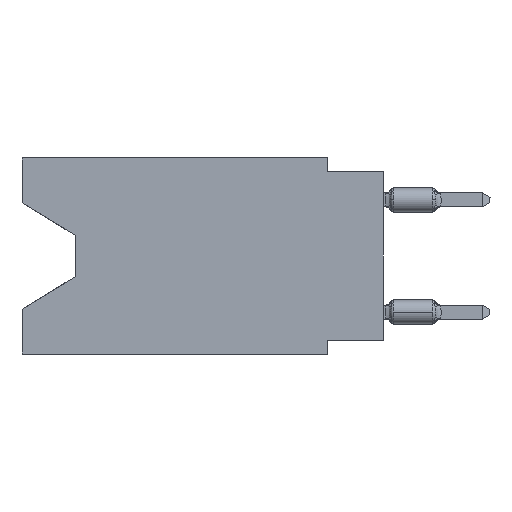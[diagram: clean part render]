
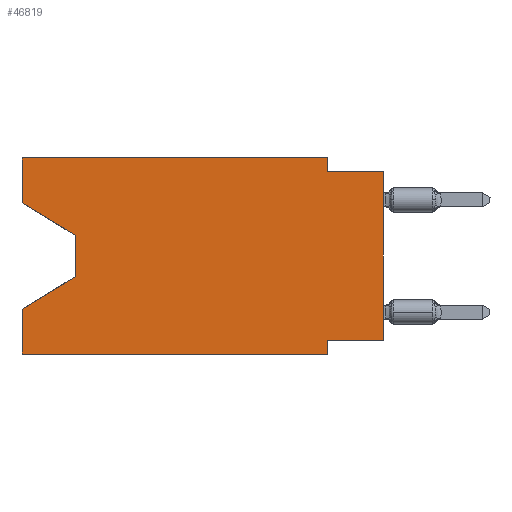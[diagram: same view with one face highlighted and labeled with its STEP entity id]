
A CAD part, left-side view. The second image highlights one B-rep face of the part: STEP entity #46819.
In plain terms, the highlighted planar face has unit normal (-1, 0, 0).
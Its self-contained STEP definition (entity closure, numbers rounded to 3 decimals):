
#721 = CARTESIAN_POINT ( 'NONE',  ( 0., 13.97, -5.385 ) ) ;
#1086 = EDGE_CURVE ( 'NONE', #20945, #19968, #5221, .T. ) ;
#1559 = CARTESIAN_POINT ( 'NONE',  ( 0., 16.383, -2.038 ) ) ;
#1664 = EDGE_CURVE ( 'NONE', #19952, #47622, #46606, .T. ) ;
#1917 = VECTOR ( 'NONE', #2793, 1000. ) ;
#2793 = DIRECTION ( 'NONE',  ( 0., 1., 0. ) ) ;
#3804 = CARTESIAN_POINT ( 'NONE',  ( 0., 16.383, 0. ) ) ;
#3839 = DIRECTION ( 'NONE',  ( 0., 0., -1. ) ) ;
#4248 = FACE_OUTER_BOUND ( 'NONE', #30074, .T. ) ;
#4250 = ORIENTED_EDGE ( 'NONE', *, *, #1664, .F. ) ;
#4386 = CARTESIAN_POINT ( 'NONE',  ( 0., 2.54, -8.255 ) ) ;
#4581 = VECTOR ( 'NONE', #15181, 1000. ) ;
#4975 = CARTESIAN_POINT ( 'NONE',  ( 0., 16.383, -2.038 ) ) ;
#5157 = ORIENTED_EDGE ( 'NONE', *, *, #45447, .F. ) ;
#5221 = LINE ( 'NONE', #34377, #26325 ) ;
#5437 = LINE ( 'NONE', #12619, #23388 ) ;
#5651 = ORIENTED_EDGE ( 'NONE', *, *, #29624, .F. ) ;
#6024 = VECTOR ( 'NONE', #39168, 1000. ) ;
#6646 = CARTESIAN_POINT ( 'NONE',  ( 0., 0., -8.255 ) ) ;
#7120 = CARTESIAN_POINT ( 'NONE',  ( 0., 16.383, -6.852 ) ) ;
#7619 = LINE ( 'NONE', #34495, #47470 ) ;
#7646 = DIRECTION ( 'NONE',  ( 0., -1., 0. ) ) ;
#9174 = LINE ( 'NONE', #24790, #21552 ) ;
#10894 = ORIENTED_EDGE ( 'NONE', *, *, #1086, .F. ) ;
#11537 = CARTESIAN_POINT ( 'NONE',  ( 0., 16.383, -8.89 ) ) ;
#12569 = DIRECTION ( 'NONE',  ( 0., -0.855, -0.519 ) ) ;
#12619 = CARTESIAN_POINT ( 'NONE',  ( 0., 16.383, -8.89 ) ) ;
#12793 = CARTESIAN_POINT ( 'NONE',  ( 0., 13.97, -5.385 ) ) ;
#13985 = ORIENTED_EDGE ( 'NONE', *, *, #17828, .T. ) ;
#15181 = DIRECTION ( 'NONE',  ( 0., 0., 1. ) ) ;
#15222 = VERTEX_POINT ( 'NONE', #11537 ) ;
#15249 = DIRECTION ( 'NONE',  ( 1., 0., 0. ) ) ;
#15275 = EDGE_CURVE ( 'NONE', #15731, #26305, #31252, .T. ) ;
#15731 = VERTEX_POINT ( 'NONE', #721 ) ;
#17105 = ORIENTED_EDGE ( 'NONE', *, *, #17678, .F. ) ;
#17678 = EDGE_CURVE ( 'NONE', #15222, #26305, #27218, .T. ) ;
#17828 = EDGE_CURVE ( 'NONE', #15222, #47622, #5437, .T. ) ;
#18212 = CARTESIAN_POINT ( 'NONE',  ( 0., 0., -0.635 ) ) ;
#18218 = ORIENTED_EDGE ( 'NONE', *, *, #15275, .T. ) ;
#18248 = ORIENTED_EDGE ( 'NONE', *, *, #48105, .F. ) ;
#19952 = VERTEX_POINT ( 'NONE', #4386 ) ;
#19968 = VERTEX_POINT ( 'NONE', #42783 ) ;
#20094 = EDGE_CURVE ( 'NONE', #20945, #23039, #44067, .T. ) ;
#20847 = CARTESIAN_POINT ( 'NONE',  ( 0., 2.54, 0. ) ) ;
#20945 = VERTEX_POINT ( 'NONE', #4975 ) ;
#21552 = VECTOR ( 'NONE', #47845, 1000. ) ;
#22370 = VECTOR ( 'NONE', #12569, 1000. ) ;
#23039 = VERTEX_POINT ( 'NONE', #49503 ) ;
#23190 = VECTOR ( 'NONE', #42718, 1000. ) ;
#23388 = VECTOR ( 'NONE', #24413, 1000. ) ;
#24151 = CARTESIAN_POINT ( 'NONE',  ( 0., 2.54, -0.635 ) ) ;
#24413 = DIRECTION ( 'NONE',  ( 0., -1., 0. ) ) ;
#24699 = LINE ( 'NONE', #20847, #35748 ) ;
#24790 = CARTESIAN_POINT ( 'NONE',  ( 0., 0., 0. ) ) ;
#24795 = VECTOR ( 'NONE', #3839, 1000. ) ;
#25985 = VERTEX_POINT ( 'NONE', #18212 ) ;
#26107 = LINE ( 'NONE', #6646, #1917 ) ;
#26305 = VERTEX_POINT ( 'NONE', #7120 ) ;
#26325 = VECTOR ( 'NONE', #38208, 1000. ) ;
#27218 = LINE ( 'NONE', #47213, #4581 ) ;
#28776 = DIRECTION ( 'NONE',  ( 0., 0., -1. ) ) ;
#29060 = VERTEX_POINT ( 'NONE', #38389 ) ;
#29624 = EDGE_CURVE ( 'NONE', #29060, #45184, #24699, .T. ) ;
#29923 = ORIENTED_EDGE ( 'NONE', *, *, #42103, .T. ) ;
#30074 = EDGE_LOOP ( 'NONE', ( #50437, #29923, #18218, #17105, #13985, #4250, #34155, #30131, #5157, #5651, #18248, #10894 ) ) ;
#30131 = ORIENTED_EDGE ( 'NONE', *, *, #48258, .T. ) ;
#30743 = CARTESIAN_POINT ( 'NONE',  ( 0., 2.54, -8.89 ) ) ;
#30910 = DIRECTION ( 'NONE',  ( 0., 0., -1. ) ) ;
#31252 = LINE ( 'NONE', #12793, #6024 ) ;
#31459 = LINE ( 'NONE', #42711, #32959 ) ;
#31907 = PLANE ( 'NONE',  #43680 ) ;
#32959 = VECTOR ( 'NONE', #7646, 1000. ) ;
#34155 = ORIENTED_EDGE ( 'NONE', *, *, #48010, .F. ) ;
#34377 = CARTESIAN_POINT ( 'NONE',  ( 0., 16.383, 0. ) ) ;
#34495 = CARTESIAN_POINT ( 'NONE',  ( 0., 13.97, -3.505 ) ) ;
#35748 = VECTOR ( 'NONE', #28776, 1000. ) ;
#37919 = CARTESIAN_POINT ( 'NONE',  ( 0., 0., -8.255 ) ) ;
#38208 = DIRECTION ( 'NONE',  ( 0., 0., 1. ) ) ;
#38389 = CARTESIAN_POINT ( 'NONE',  ( 0., 2.54, 0. ) ) ;
#39168 = DIRECTION ( 'NONE',  ( 0., 0.855, -0.519 ) ) ;
#42103 = EDGE_CURVE ( 'NONE', #23039, #15731, #7619, .T. ) ;
#42711 = CARTESIAN_POINT ( 'NONE',  ( 0., 0., -0.635 ) ) ;
#42718 = DIRECTION ( 'NONE',  ( 0., -1., 0. ) ) ;
#42783 = CARTESIAN_POINT ( 'NONE',  ( 0., 16.383, 0. ) ) ;
#43680 = AXIS2_PLACEMENT_3D ( 'NONE', #46495, #15249, #47275 ) ;
#44067 = LINE ( 'NONE', #1559, #22370 ) ;
#45184 = VERTEX_POINT ( 'NONE', #24151 ) ;
#45447 = EDGE_CURVE ( 'NONE', #45184, #25985, #31459, .T. ) ;
#46495 = CARTESIAN_POINT ( 'NONE',  ( 0., 16.383, 0. ) ) ;
#46606 = LINE ( 'NONE', #50198, #24795 ) ;
#46819 = ADVANCED_FACE ( 'NONE', ( #4248 ), #31907, .F. ) ;
#46829 = LINE ( 'NONE', #3804, #23190 ) ;
#47213 = CARTESIAN_POINT ( 'NONE',  ( 0., 16.383, 0. ) ) ;
#47275 = DIRECTION ( 'NONE',  ( 0., 0., -1. ) ) ;
#47470 = VECTOR ( 'NONE', #30910, 1000. ) ;
#47622 = VERTEX_POINT ( 'NONE', #30743 ) ;
#47845 = DIRECTION ( 'NONE',  ( 0., 0., 1. ) ) ;
#48010 = EDGE_CURVE ( 'NONE', #48724, #19952, #26107, .T. ) ;
#48105 = EDGE_CURVE ( 'NONE', #19968, #29060, #46829, .T. ) ;
#48258 = EDGE_CURVE ( 'NONE', #48724, #25985, #9174, .T. ) ;
#48724 = VERTEX_POINT ( 'NONE', #37919 ) ;
#49503 = CARTESIAN_POINT ( 'NONE',  ( 0., 13.97, -3.505 ) ) ;
#50198 = CARTESIAN_POINT ( 'NONE',  ( 0., 2.54, -8.89 ) ) ;
#50437 = ORIENTED_EDGE ( 'NONE', *, *, #20094, .T. ) ;
